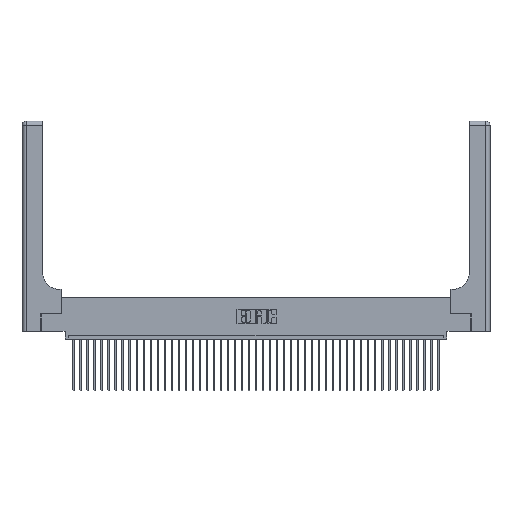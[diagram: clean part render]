
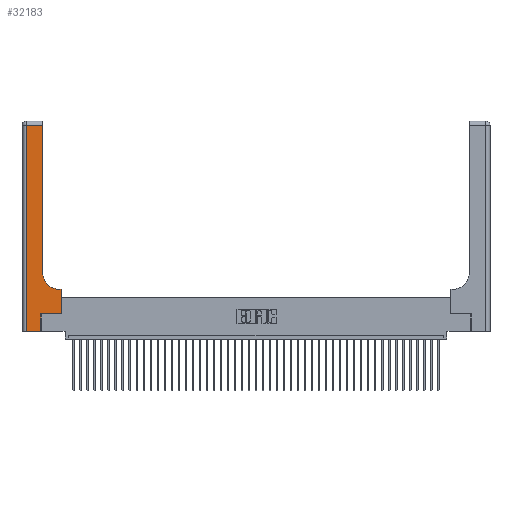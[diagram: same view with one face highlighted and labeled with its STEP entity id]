
A CAD part, top view. The second image highlights one B-rep face of the part: STEP entity #32183.
In plain terms, the highlighted planar face has unit normal (0, 0, 1).
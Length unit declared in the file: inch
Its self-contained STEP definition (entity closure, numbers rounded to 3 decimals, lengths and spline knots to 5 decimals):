
#484 = CARTESIAN_POINT ( 'NONE',  ( 0.5585, 0.25, 0.37 ) ) ;
#599 = VERTEX_POINT ( 'NONE', #1080 ) ;
#864 = EDGE_CURVE ( 'NONE', #21662, #4148, #4939, .T. ) ;
#1080 = CARTESIAN_POINT ( 'NONE',  ( 0.5415, 0.6, 0.37 ) ) ;
#1344 = CARTESIAN_POINT ( 'NONE',  ( 0.06, 2.94, 0.37 ) ) ;
#1845 = VECTOR ( 'NONE', #22119, 39.37008 ) ;
#2843 = VERTEX_POINT ( 'NONE', #20600 ) ;
#4050 = CARTESIAN_POINT ( 'NONE',  ( 0.2915, 0.85, 0.37 ) ) ;
#4148 = VERTEX_POINT ( 'NONE', #37848 ) ;
#4939 = LINE ( 'NONE', #29387, #35076 ) ;
#5930 = LINE ( 'NONE', #39892, #32381 ) ;
#7424 = EDGE_CURVE ( 'NONE', #15155, #10897, #27576, .T. ) ;
#7770 = ORIENTED_EDGE ( 'NONE', *, *, #864, .T. ) ;
#8274 = VECTOR ( 'NONE', #41993, 39.37008 ) ;
#9387 = CARTESIAN_POINT ( 'NONE',  ( 0.269, 0., 0.37 ) ) ;
#10308 = DIRECTION ( 'NONE',  ( 0., 0., -1. ) ) ;
#10348 = LINE ( 'NONE', #42300, #1845 ) ;
#10506 = CARTESIAN_POINT ( 'NONE',  ( 0.2915, 2.94, 0.37 ) ) ;
#10563 = CARTESIAN_POINT ( 'NONE',  ( 0.5415, 0.85, 0.37 ) ) ;
#10829 = DIRECTION ( 'NONE',  ( 0., 1., 0. ) ) ;
#10897 = VERTEX_POINT ( 'NONE', #1344 ) ;
#11041 = CARTESIAN_POINT ( 'NONE',  ( 0., 0., 0.37 ) ) ;
#11991 = VERTEX_POINT ( 'NONE', #28746 ) ;
#13001 = EDGE_CURVE ( 'NONE', #10897, #11991, #5930, .T. ) ;
#13788 = EDGE_LOOP ( 'NONE', ( #39403, #16273, #42612, #33332, #7770, #37830, #39241, #25784, #32753 ) ) ;
#13790 = EDGE_CURVE ( 'NONE', #2843, #599, #10348, .T. ) ;
#14087 = AXIS2_PLACEMENT_3D ( 'NONE', #27186, #10308, #14164 ) ;
#14164 = DIRECTION ( 'NONE',  ( -1., 0., 0. ) ) ;
#15155 = VERTEX_POINT ( 'NONE', #10506 ) ;
#16273 = ORIENTED_EDGE ( 'NONE', *, *, #7424, .T. ) ;
#18470 = CARTESIAN_POINT ( 'NONE',  ( 0.269, 0.25, 0.37 ) ) ;
#19273 = VECTOR ( 'NONE', #10829, 39.37008 ) ;
#20600 = CARTESIAN_POINT ( 'NONE',  ( 0.5585, 0.6, 0.37 ) ) ;
#20620 = CARTESIAN_POINT ( 'NONE',  ( 0.2915, 3., 0.37 ) ) ;
#21484 = CARTESIAN_POINT ( 'NONE',  ( 0., 2.94, 0.37 ) ) ;
#21592 = VERTEX_POINT ( 'NONE', #34693 ) ;
#21662 = VERTEX_POINT ( 'NONE', #9387 ) ;
#22086 = LINE ( 'NONE', #18470, #8274 ) ;
#22119 = DIRECTION ( 'NONE',  ( -1., 0., 0. ) ) ;
#23093 = EDGE_CURVE ( 'NONE', #11991, #21662, #35635, .T. ) ;
#25784 = ORIENTED_EDGE ( 'NONE', *, *, #13790, .T. ) ;
#27186 = CARTESIAN_POINT ( 'NONE',  ( 0., 3., 0.37 ) ) ;
#27576 = LINE ( 'NONE', #21484, #31245 ) ;
#28102 = EDGE_CURVE ( 'NONE', #599, #35365, #35949, .T. ) ;
#28270 = DIRECTION ( 'NONE',  ( -1., 0., 0. ) ) ;
#28746 = CARTESIAN_POINT ( 'NONE',  ( 0.06, 0., 0.37 ) ) ;
#29387 = CARTESIAN_POINT ( 'NONE',  ( 0.269, 0., 0.37 ) ) ;
#29896 = VECTOR ( 'NONE', #42728, 39.37008 ) ;
#30832 = VECTOR ( 'NONE', #41211, 39.37008 ) ;
#31245 = VECTOR ( 'NONE', #28270, 39.37008 ) ;
#31956 = DIRECTION ( 'NONE',  ( 0., 0., -1. ) ) ;
#32183 = ADVANCED_FACE ( 'NONE', ( #34512 ), #37157, .F. ) ;
#32381 = VECTOR ( 'NONE', #35328, 39.37008 ) ;
#32753 = ORIENTED_EDGE ( 'NONE', *, *, #28102, .T. ) ;
#32952 = LINE ( 'NONE', #20620, #30832 ) ;
#33209 = DIRECTION ( 'NONE',  ( 0., 1., 0. ) ) ;
#33332 = ORIENTED_EDGE ( 'NONE', *, *, #23093, .T. ) ;
#34512 = FACE_OUTER_BOUND ( 'NONE', #13788, .T. ) ;
#34693 = CARTESIAN_POINT ( 'NONE',  ( 0.5585, 0.25, 0.37 ) ) ;
#35076 = VECTOR ( 'NONE', #33209, 39.37008 ) ;
#35207 = DIRECTION ( 'NONE',  ( 1., 0., 0. ) ) ;
#35328 = DIRECTION ( 'NONE',  ( 0., -1., 0. ) ) ;
#35365 = VERTEX_POINT ( 'NONE', #4050 ) ;
#35635 = LINE ( 'NONE', #11041, #29896 ) ;
#35949 = CIRCLE ( 'NONE', #41376, 0.25 ) ;
#36034 = EDGE_CURVE ( 'NONE', #35365, #15155, #32952, .T. ) ;
#36048 = EDGE_CURVE ( 'NONE', #21592, #2843, #40790, .T. ) ;
#37157 = PLANE ( 'NONE',  #14087 ) ;
#37830 = ORIENTED_EDGE ( 'NONE', *, *, #40211, .T. ) ;
#37848 = CARTESIAN_POINT ( 'NONE',  ( 0.269, 0.25, 0.37 ) ) ;
#39241 = ORIENTED_EDGE ( 'NONE', *, *, #36048, .T. ) ;
#39403 = ORIENTED_EDGE ( 'NONE', *, *, #36034, .T. ) ;
#39892 = CARTESIAN_POINT ( 'NONE',  ( 0.06, 3., 0.37 ) ) ;
#40211 = EDGE_CURVE ( 'NONE', #4148, #21592, #22086, .T. ) ;
#40790 = LINE ( 'NONE', #484, #19273 ) ;
#41211 = DIRECTION ( 'NONE',  ( 0., 1., 0. ) ) ;
#41376 = AXIS2_PLACEMENT_3D ( 'NONE', #10563, #31956, #35207 ) ;
#41993 = DIRECTION ( 'NONE',  ( 1., 0., 0. ) ) ;
#42300 = CARTESIAN_POINT ( 'NONE',  ( 0.2915, 0.6, 0.37 ) ) ;
#42612 = ORIENTED_EDGE ( 'NONE', *, *, #13001, .T. ) ;
#42728 = DIRECTION ( 'NONE',  ( 1., 0., 0. ) ) ;
